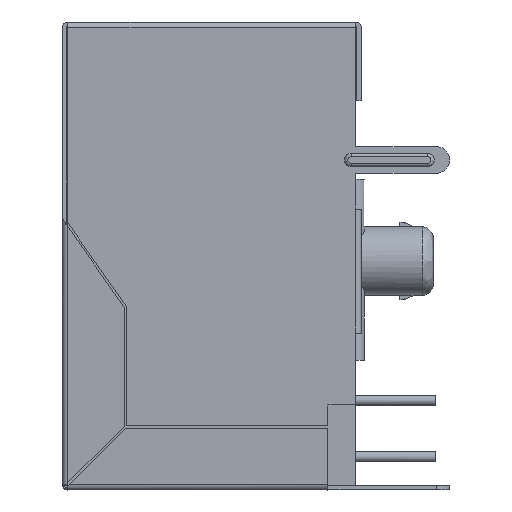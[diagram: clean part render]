
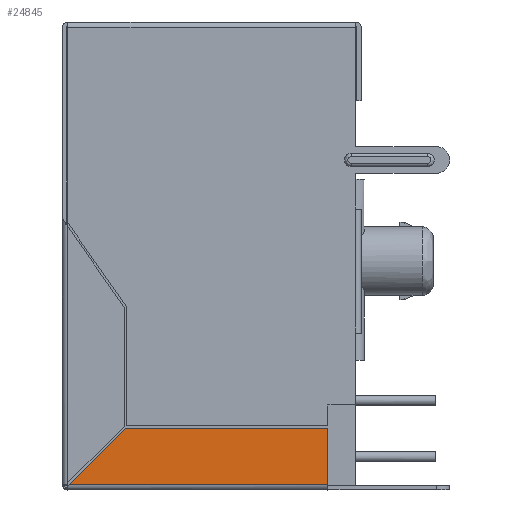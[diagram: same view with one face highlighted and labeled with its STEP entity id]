
A CAD part, left-side view. The second image highlights one B-rep face of the part: STEP entity #24845.
In plain terms, the highlighted planar face has unit normal (-1, 0, 0).
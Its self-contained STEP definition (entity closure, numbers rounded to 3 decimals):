
#3350 = CARTESIAN_POINT ( 'NONE',  ( -29.45, -11.75, -18.97 ) ) ;
#4750 = EDGE_CURVE ( 'NONE', #5392, #15816, #26590, .T. ) ;
#4761 = EDGE_CURVE ( 'NONE', #15816, #10558, #28403, .T. ) ;
#5051 = DIRECTION ( 'NONE',  ( 0., 0., 1. ) ) ;
#5392 = VERTEX_POINT ( 'NONE', #26183 ) ;
#6900 = VECTOR ( 'NONE', #12851, 1000. ) ;
#7239 = EDGE_LOOP ( 'NONE', ( #27113, #13133, #21480, #22055 ) ) ;
#10558 = VERTEX_POINT ( 'NONE', #21381 ) ;
#10673 = PLANE ( 'NONE',  #14764 ) ;
#11087 = FACE_OUTER_BOUND ( 'NONE', #7239, .T. ) ;
#11666 = LINE ( 'NONE', #3350, #30907 ) ;
#12244 = EDGE_CURVE ( 'NONE', #23697, #5392, #14515, .T. ) ;
#12851 = DIRECTION ( 'NONE',  ( 0., 1., 0. ) ) ;
#13133 = ORIENTED_EDGE ( 'NONE', *, *, #12244, .T. ) ;
#13346 = EDGE_CURVE ( 'NONE', #23697, #10558, #11666, .T. ) ;
#14034 = CARTESIAN_POINT ( 'NONE',  ( -29.45, -1.241, -19.469 ) ) ;
#14515 = LINE ( 'NONE', #32640, #6900 ) ;
#14764 = AXIS2_PLACEMENT_3D ( 'NONE', #30721, #25316, #5051 ) ;
#15816 = VERTEX_POINT ( 'NONE', #28498 ) ;
#16651 = DIRECTION ( 'NONE',  ( 0., 0.707, -0.707 ) ) ;
#16897 = DIRECTION ( 'NONE',  ( 0., -1., 0. ) ) ;
#17824 = DIRECTION ( 'NONE',  ( 0., 0., -1. ) ) ;
#21381 = CARTESIAN_POINT ( 'NONE',  ( -29.45, -11.75, -20.64 ) ) ;
#21480 = ORIENTED_EDGE ( 'NONE', *, *, #4750, .T. ) ;
#22055 = ORIENTED_EDGE ( 'NONE', *, *, #4761, .T. ) ;
#23697 = VERTEX_POINT ( 'NONE', #24083 ) ;
#24083 = CARTESIAN_POINT ( 'NONE',  ( -29.45, -11.75, -18.09 ) ) ;
#24845 = ADVANCED_FACE ( 'NONE', ( #11087 ), #10673, .T. ) ;
#25316 = DIRECTION ( 'NONE',  ( -1., 0., 0. ) ) ;
#26183 = CARTESIAN_POINT ( 'NONE',  ( -29.45, -2.621, -18.09 ) ) ;
#26590 = LINE ( 'NONE', #14034, #31525 ) ;
#27113 = ORIENTED_EDGE ( 'NONE', *, *, #13346, .F. ) ;
#27930 = VECTOR ( 'NONE', #16897, 1000. ) ;
#28214 = CARTESIAN_POINT ( 'NONE',  ( -29.45, -8.626, -20.64 ) ) ;
#28403 = LINE ( 'NONE', #28214, #27930 ) ;
#28498 = CARTESIAN_POINT ( 'NONE',  ( -29.45, -0.071, -20.64 ) ) ;
#30721 = CARTESIAN_POINT ( 'NONE',  ( -29.45, -17.598, -21.053 ) ) ;
#30907 = VECTOR ( 'NONE', #17824, 1000. ) ;
#31525 = VECTOR ( 'NONE', #16651, 1000. ) ;
#32640 = CARTESIAN_POINT ( 'NONE',  ( -29.45, -7.185, -18.09 ) ) ;
